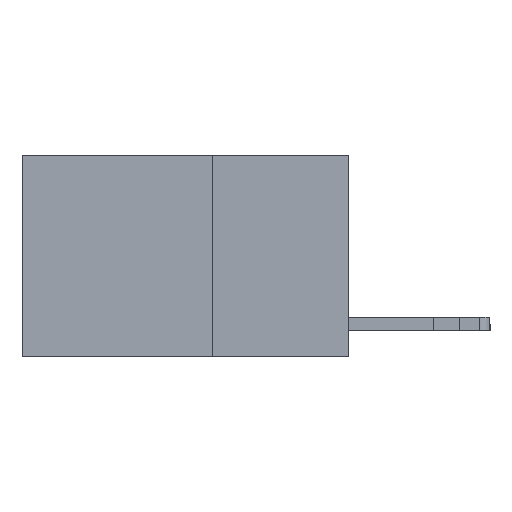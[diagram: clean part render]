
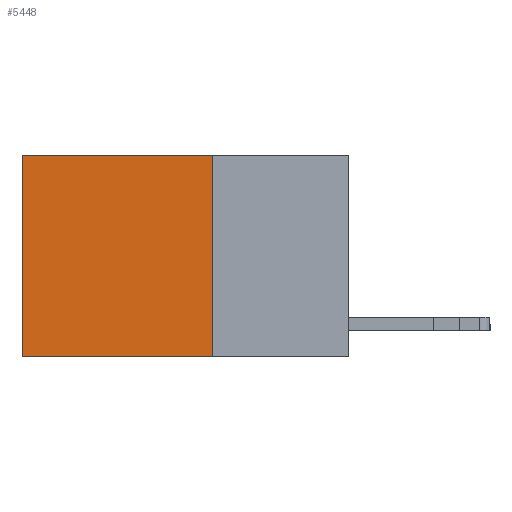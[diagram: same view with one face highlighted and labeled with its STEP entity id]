
A CAD part, left-side view. The second image highlights one B-rep face of the part: STEP entity #5448.
In plain terms, the highlighted planar face has unit normal (-1, 0, 0).
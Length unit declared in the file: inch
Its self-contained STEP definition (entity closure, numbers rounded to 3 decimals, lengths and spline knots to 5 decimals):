
#176 = LINE ( 'NONE', #8323, #20253 ) ;
#178 = VECTOR ( 'NONE', #2366, 39.37008 ) ;
#1384 = DIRECTION ( 'NONE',  ( 1., 0., 0. ) ) ;
#2366 = DIRECTION ( 'NONE',  ( 0., 1., 0. ) ) ;
#2710 = EDGE_CURVE ( 'NONE', #10347, #12723, #176, .T. ) ;
#2834 = DIRECTION ( 'NONE',  ( 0., 0., -1. ) ) ;
#2892 = EDGE_CURVE ( 'NONE', #12723, #14519, #6707, .T. ) ;
#4606 = ORIENTED_EDGE ( 'NONE', *, *, #2710, .T. ) ;
#5448 = ADVANCED_FACE ( 'NONE', ( #11540 ), #16107, .F. ) ;
#6018 = VECTOR ( 'NONE', #2834, 39.37008 ) ;
#6456 = CARTESIAN_POINT ( 'NONE',  ( 0.2625, 0.25, 0. ) ) ;
#6707 = LINE ( 'NONE', #14876, #8238 ) ;
#7705 = CARTESIAN_POINT ( 'NONE',  ( 0.2625, 0.25, 0. ) ) ;
#8238 = VECTOR ( 'NONE', #17272, 39.37008 ) ;
#8323 = CARTESIAN_POINT ( 'NONE',  ( 0.2625, 0.25, 0. ) ) ;
#9535 = DIRECTION ( 'NONE',  ( 0., 0., -1. ) ) ;
#9822 = ORIENTED_EDGE ( 'NONE', *, *, #2892, .T. ) ;
#10097 = CARTESIAN_POINT ( 'NONE',  ( 0.2625, 0.6, -0.37 ) ) ;
#10255 = LINE ( 'NONE', #20842, #178 ) ;
#10347 = VERTEX_POINT ( 'NONE', #7705 ) ;
#11525 = CARTESIAN_POINT ( 'NONE',  ( 0.2625, 0.25, -0.37 ) ) ;
#11540 = FACE_OUTER_BOUND ( 'NONE', #23689, .T. ) ;
#11786 = ORIENTED_EDGE ( 'NONE', *, *, #23247, .F. ) ;
#12723 = VERTEX_POINT ( 'NONE', #13512 ) ;
#12849 = LINE ( 'NONE', #6456, #6018 ) ;
#13512 = CARTESIAN_POINT ( 'NONE',  ( 0.2625, 0.6, 0. ) ) ;
#13526 = VERTEX_POINT ( 'NONE', #11525 ) ;
#14346 = DIRECTION ( 'NONE',  ( 0., 1., 0. ) ) ;
#14519 = VERTEX_POINT ( 'NONE', #10097 ) ;
#14816 = ORIENTED_EDGE ( 'NONE', *, *, #21050, .F. ) ;
#14876 = CARTESIAN_POINT ( 'NONE',  ( 0.2625, 0.6, 0. ) ) ;
#16107 = PLANE ( 'NONE',  #23275 ) ;
#17272 = DIRECTION ( 'NONE',  ( 0., 0., -1. ) ) ;
#20253 = VECTOR ( 'NONE', #14346, 39.37008 ) ;
#20842 = CARTESIAN_POINT ( 'NONE',  ( 0.2625, 0.25, -0.37 ) ) ;
#21050 = EDGE_CURVE ( 'NONE', #10347, #13526, #12849, .T. ) ;
#23247 = EDGE_CURVE ( 'NONE', #13526, #14519, #10255, .T. ) ;
#23275 = AXIS2_PLACEMENT_3D ( 'NONE', #24314, #1384, #9535 ) ;
#23689 = EDGE_LOOP ( 'NONE', ( #9822, #11786, #14816, #4606 ) ) ;
#24314 = CARTESIAN_POINT ( 'NONE',  ( 0.2625, 0.25, 0. ) ) ;
